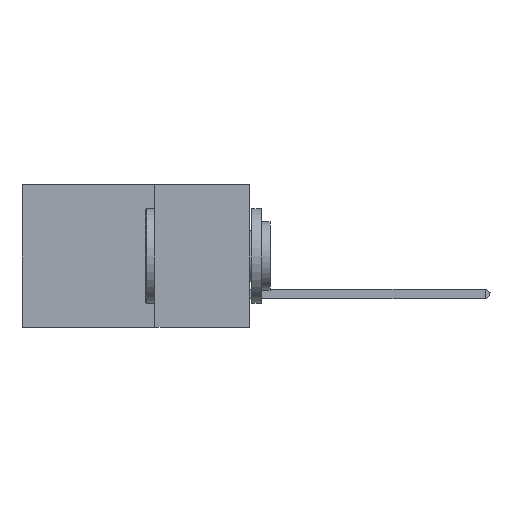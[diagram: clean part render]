
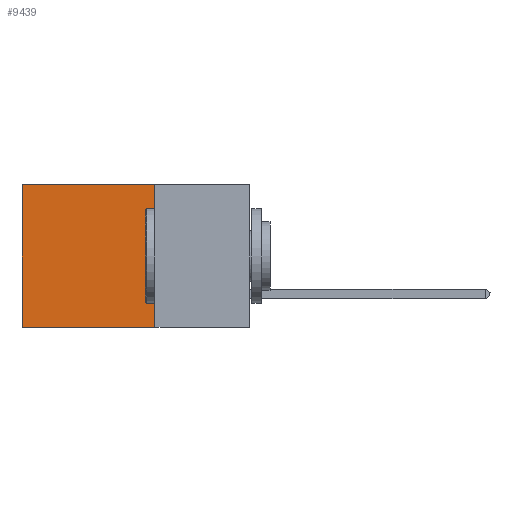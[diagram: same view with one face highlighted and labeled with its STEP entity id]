
A CAD part, left-side view. The second image highlights one B-rep face of the part: STEP entity #9439.
In plain terms, the highlighted planar face has unit normal (-1, 0, 0).
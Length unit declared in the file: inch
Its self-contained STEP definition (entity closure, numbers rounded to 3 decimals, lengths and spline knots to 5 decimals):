
#23 = VERTEX_POINT ( 'NONE', #5875 ) ;
#169 = PLANE ( 'NONE',  #15721 ) ;
#418 = EDGE_CURVE ( 'NONE', #21039, #11655, #10641, .T. ) ;
#946 = EDGE_CURVE ( 'NONE', #19456, #21039, #15028, .T. ) ;
#3241 = CARTESIAN_POINT ( 'NONE',  ( 0.2875, 0.25, -0.375 ) ) ;
#4706 = EDGE_CURVE ( 'NONE', #23, #11655, #16827, .T. ) ;
#5785 = CARTESIAN_POINT ( 'NONE',  ( 0.2875, 0.25, 0. ) ) ;
#5875 = CARTESIAN_POINT ( 'NONE',  ( 0.2875, 0.25, -0.375 ) ) ;
#6292 = EDGE_CURVE ( 'NONE', #19456, #23, #19923, .T. ) ;
#6704 = CARTESIAN_POINT ( 'NONE',  ( 0.2875, 0.25, 0. ) ) ;
#6725 = CARTESIAN_POINT ( 'NONE',  ( 0.2875, 0.6, -0.375 ) ) ;
#7266 = ORIENTED_EDGE ( 'NONE', *, *, #946, .T. ) ;
#7737 = VECTOR ( 'NONE', #14849, 39.37008 ) ;
#9439 = ADVANCED_FACE ( 'NONE', ( #16980 ), #169, .F. ) ;
#9448 = CARTESIAN_POINT ( 'NONE',  ( 0.2875, 0.6, 0. ) ) ;
#10641 = LINE ( 'NONE', #6725, #16589 ) ;
#11655 = VERTEX_POINT ( 'NONE', #12430 ) ;
#11724 = DIRECTION ( 'NONE',  ( 0., 0., -1. ) ) ;
#11800 = CARTESIAN_POINT ( 'NONE',  ( 0.2875, 0.25, -0.375 ) ) ;
#12002 = DIRECTION ( 'NONE',  ( 0., 1., 0. ) ) ;
#12140 = ORIENTED_EDGE ( 'NONE', *, *, #4706, .F. ) ;
#12430 = CARTESIAN_POINT ( 'NONE',  ( 0.2875, 0.6, -0.375 ) ) ;
#13370 = DIRECTION ( 'NONE',  ( 0., 0., -1. ) ) ;
#13530 = DIRECTION ( 'NONE',  ( 1., 0., 0. ) ) ;
#14849 = DIRECTION ( 'NONE',  ( 0., 1., 0. ) ) ;
#15028 = LINE ( 'NONE', #6704, #15804 ) ;
#15132 = DIRECTION ( 'NONE',  ( 0., 0., -1. ) ) ;
#15721 = AXIS2_PLACEMENT_3D ( 'NONE', #11800, #13530, #15132 ) ;
#15804 = VECTOR ( 'NONE', #12002, 39.37008 ) ;
#16589 = VECTOR ( 'NONE', #11724, 39.37008 ) ;
#16707 = CARTESIAN_POINT ( 'NONE',  ( 0.2875, 0.25, -0.375 ) ) ;
#16827 = LINE ( 'NONE', #3241, #7737 ) ;
#16958 = ORIENTED_EDGE ( 'NONE', *, *, #418, .T. ) ;
#16980 = FACE_OUTER_BOUND ( 'NONE', #17740, .T. ) ;
#17740 = EDGE_LOOP ( 'NONE', ( #16958, #12140, #18315, #7266 ) ) ;
#18315 = ORIENTED_EDGE ( 'NONE', *, *, #6292, .F. ) ;
#18617 = VECTOR ( 'NONE', #13370, 39.37008 ) ;
#19456 = VERTEX_POINT ( 'NONE', #5785 ) ;
#19923 = LINE ( 'NONE', #16707, #18617 ) ;
#21039 = VERTEX_POINT ( 'NONE', #9448 ) ;
